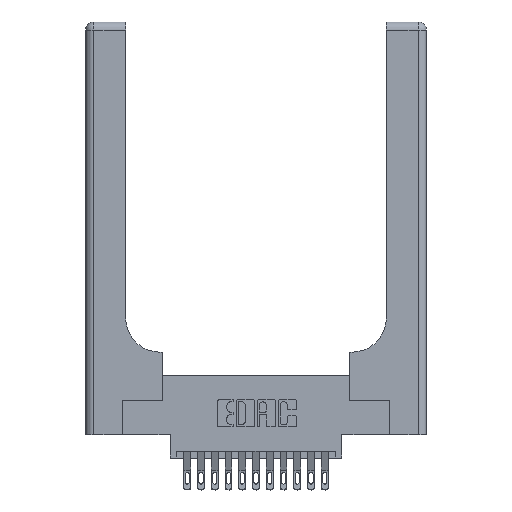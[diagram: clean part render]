
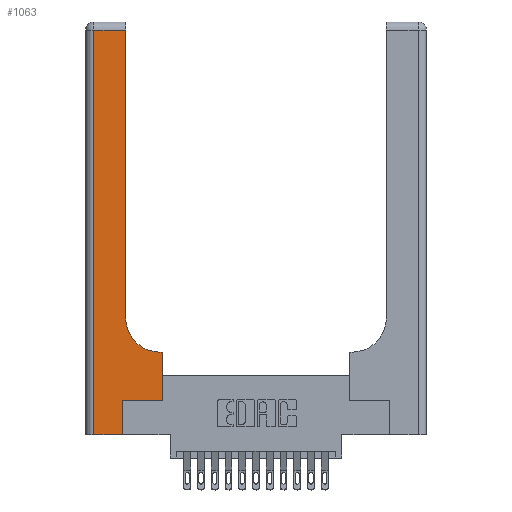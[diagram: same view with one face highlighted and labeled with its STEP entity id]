
A CAD part, top view. The second image highlights one B-rep face of the part: STEP entity #1063.
In plain terms, the highlighted planar face has unit normal (0, 0, 1).
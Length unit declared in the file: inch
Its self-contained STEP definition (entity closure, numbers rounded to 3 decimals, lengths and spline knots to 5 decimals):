
#341 = VERTEX_POINT ( 'NONE', #1619 ) ;
#371 = CARTESIAN_POINT ( 'NONE',  ( 0.5585, 0.25, 0.37 ) ) ;
#802 = LINE ( 'NONE', #6385, #15180 ) ;
#823 = EDGE_CURVE ( 'NONE', #16624, #10486, #802, .T. ) ;
#850 = CARTESIAN_POINT ( 'NONE',  ( 0.269, 0., 0.37 ) ) ;
#854 = VERTEX_POINT ( 'NONE', #6060 ) ;
#1063 = ADVANCED_FACE ( 'NONE', ( #15385 ), #2132, .F. ) ;
#1125 = VERTEX_POINT ( 'NONE', #850 ) ;
#1379 = CARTESIAN_POINT ( 'NONE',  ( 0., 0., 0.37 ) ) ;
#1619 = CARTESIAN_POINT ( 'NONE',  ( 0.06, 0., 0.37 ) ) ;
#1918 = DIRECTION ( 'NONE',  ( -1., 0., 0. ) ) ;
#1999 = CARTESIAN_POINT ( 'NONE',  ( 0.2915, 0.6, 0.37 ) ) ;
#2025 = DIRECTION ( 'NONE',  ( -1., 0., 0. ) ) ;
#2044 = DIRECTION ( 'NONE',  ( 0., 0., -1. ) ) ;
#2126 = VECTOR ( 'NONE', #1918, 39.37008 ) ;
#2132 = PLANE ( 'NONE',  #4113 ) ;
#2143 = CARTESIAN_POINT ( 'NONE',  ( 0.2915, 0.85, 0.37 ) ) ;
#2218 = CARTESIAN_POINT ( 'NONE',  ( 0., 3., 0.37 ) ) ;
#2655 = ORIENTED_EDGE ( 'NONE', *, *, #12169, .T. ) ;
#3247 = LINE ( 'NONE', #1379, #6759 ) ;
#3262 = CARTESIAN_POINT ( 'NONE',  ( 0.269, 0., 0.37 ) ) ;
#3719 = EDGE_CURVE ( 'NONE', #854, #17569, #13549, .T. ) ;
#3768 = CIRCLE ( 'NONE', #13059, 0.25 ) ;
#3912 = ORIENTED_EDGE ( 'NONE', *, *, #18257, .T. ) ;
#4000 = CARTESIAN_POINT ( 'NONE',  ( 0.5415, 0.85, 0.37 ) ) ;
#4082 = LINE ( 'NONE', #8064, #11304 ) ;
#4113 = AXIS2_PLACEMENT_3D ( 'NONE', #2218, #2044, #2025 ) ;
#4143 = ORIENTED_EDGE ( 'NONE', *, *, #10127, .T. ) ;
#4351 = DIRECTION ( 'NONE',  ( 1., 0., 0. ) ) ;
#4421 = LINE ( 'NONE', #3262, #8781 ) ;
#4554 = ORIENTED_EDGE ( 'NONE', *, *, #11657, .T. ) ;
#4616 = CARTESIAN_POINT ( 'NONE',  ( 0.269, 0.25, 0.37 ) ) ;
#4783 = LINE ( 'NONE', #4616, #11930 ) ;
#5542 = DIRECTION ( 'NONE',  ( 1., 0., 0. ) ) ;
#6060 = CARTESIAN_POINT ( 'NONE',  ( 0.5585, 0.6, 0.37 ) ) ;
#6385 = CARTESIAN_POINT ( 'NONE',  ( 0.2915, 3., 0.37 ) ) ;
#6442 = DIRECTION ( 'NONE',  ( 0., 1., 0. ) ) ;
#6759 = VECTOR ( 'NONE', #4351, 39.37008 ) ;
#7147 = CARTESIAN_POINT ( 'NONE',  ( 0.2915, 2.94, 0.37 ) ) ;
#7404 = ORIENTED_EDGE ( 'NONE', *, *, #823, .T. ) ;
#7514 = EDGE_CURVE ( 'NONE', #16284, #9554, #4783, .T. ) ;
#8064 = CARTESIAN_POINT ( 'NONE',  ( 0.5585, 0.25, 0.37 ) ) ;
#8583 = LINE ( 'NONE', #11288, #15516 ) ;
#8781 = VECTOR ( 'NONE', #13244, 39.37008 ) ;
#8822 = CARTESIAN_POINT ( 'NONE',  ( 0.5415, 0.6, 0.37 ) ) ;
#8824 = CARTESIAN_POINT ( 'NONE',  ( 0.269, 0.25, 0.37 ) ) ;
#9047 = ORIENTED_EDGE ( 'NONE', *, *, #3719, .T. ) ;
#9088 = ORIENTED_EDGE ( 'NONE', *, *, #7514, .T. ) ;
#9554 = VERTEX_POINT ( 'NONE', #371 ) ;
#9825 = ORIENTED_EDGE ( 'NONE', *, *, #14999, .T. ) ;
#9890 = EDGE_CURVE ( 'NONE', #13060, #341, #8583, .T. ) ;
#10127 = EDGE_CURVE ( 'NONE', #1125, #16284, #4421, .T. ) ;
#10486 = VERTEX_POINT ( 'NONE', #7147 ) ;
#11288 = CARTESIAN_POINT ( 'NONE',  ( 0.06, 3., 0.37 ) ) ;
#11304 = VECTOR ( 'NONE', #14982, 39.37008 ) ;
#11657 = EDGE_CURVE ( 'NONE', #341, #1125, #3247, .T. ) ;
#11812 = DIRECTION ( 'NONE',  ( 1., 0., 0. ) ) ;
#11839 = CARTESIAN_POINT ( 'NONE',  ( 0.06, 2.94, 0.37 ) ) ;
#11930 = VECTOR ( 'NONE', #11812, 39.37008 ) ;
#12169 = EDGE_CURVE ( 'NONE', #10486, #13060, #12822, .T. ) ;
#12822 = LINE ( 'NONE', #13542, #16547 ) ;
#13059 = AXIS2_PLACEMENT_3D ( 'NONE', #4000, #13956, #5542 ) ;
#13060 = VERTEX_POINT ( 'NONE', #11839 ) ;
#13244 = DIRECTION ( 'NONE',  ( 0., 1., 0. ) ) ;
#13542 = CARTESIAN_POINT ( 'NONE',  ( 0., 2.94, 0.37 ) ) ;
#13549 = LINE ( 'NONE', #1999, #2126 ) ;
#13956 = DIRECTION ( 'NONE',  ( 0., 0., -1. ) ) ;
#14982 = DIRECTION ( 'NONE',  ( 0., 1., 0. ) ) ;
#14999 = EDGE_CURVE ( 'NONE', #17569, #16624, #3768, .T. ) ;
#15180 = VECTOR ( 'NONE', #6442, 39.37008 ) ;
#15342 = EDGE_LOOP ( 'NONE', ( #7404, #2655, #17646, #4554, #4143, #9088, #3912, #9047, #9825 ) ) ;
#15385 = FACE_OUTER_BOUND ( 'NONE', #15342, .T. ) ;
#15516 = VECTOR ( 'NONE', #18112, 39.37008 ) ;
#16284 = VERTEX_POINT ( 'NONE', #8824 ) ;
#16547 = VECTOR ( 'NONE', #17624, 39.37008 ) ;
#16624 = VERTEX_POINT ( 'NONE', #2143 ) ;
#17569 = VERTEX_POINT ( 'NONE', #8822 ) ;
#17624 = DIRECTION ( 'NONE',  ( -1., 0., 0. ) ) ;
#17646 = ORIENTED_EDGE ( 'NONE', *, *, #9890, .T. ) ;
#18112 = DIRECTION ( 'NONE',  ( 0., -1., 0. ) ) ;
#18257 = EDGE_CURVE ( 'NONE', #9554, #854, #4082, .T. ) ;
